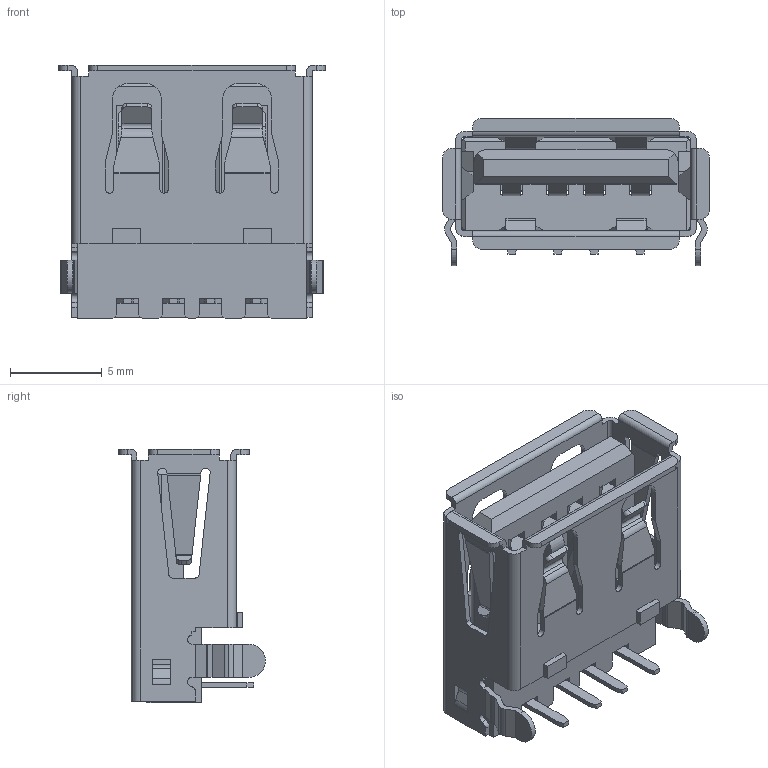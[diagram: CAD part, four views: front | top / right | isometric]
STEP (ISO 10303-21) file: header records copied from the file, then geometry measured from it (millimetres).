
FILE_DESCRIPTION (( 'STEP AP214' ), '1' );
FILE_NAME ('690G104-153-021.STEP', '2021-01-14T13:17:50', ( '' ), ( '' ), 'SwSTEP 2.0', 'SolidWorks 2020', '' );
FILE_SCHEMA (( 'AUTOMOTIVE_DESIGN' ));
Length unit declared in the file: millimetre
Products named in the file (4): Contact 690G104-X53-02X; Insulator 690G104-X53-02X_Black; Shell 690G104-X53-02X; 690G104-153-021
Assembly tree (6 placements, depth 2):
  690G104-153-021
    Insulator 690G104-X53-02X_Black
    Contact 690G104-X53-02X  x4
    Shell 690G104-X53-02X
Bounding box: 14.5 x 8 x 13.78 mm (x, y, z)
Volume: 412.6 mm3; surface area: 1755 mm2
Topology: 6 solids, 6 shells, 743 faces, 2147 edges, 1406 vertices
Faces by surface type: plane 561, cylinder 166, bspline 16
Entity records: 19171 total; most frequent: CARTESIAN_POINT 3894, ORIENTED_EDGE 3304, DIRECTION 2969, EDGE_CURVE 1652, LINE 1347, VECTOR 1347, VERTEX_POINT 1076, AXIS2_PLACEMENT_3D 811
